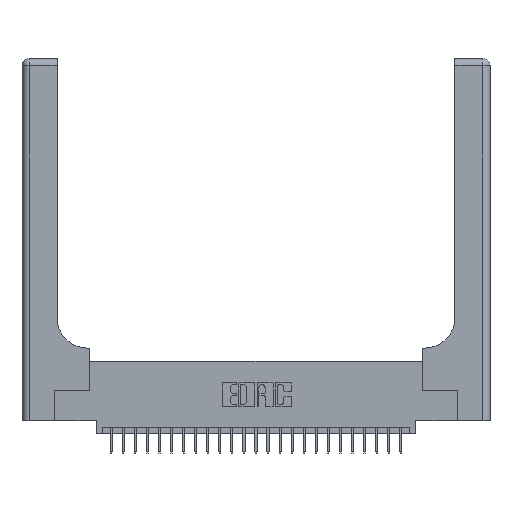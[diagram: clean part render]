
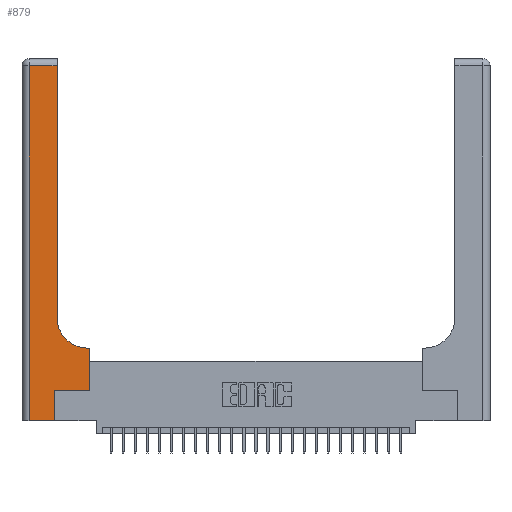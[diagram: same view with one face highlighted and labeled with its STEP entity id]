
A CAD part, top view. The second image highlights one B-rep face of the part: STEP entity #879.
In plain terms, the highlighted planar face has unit normal (0, 0, 1).
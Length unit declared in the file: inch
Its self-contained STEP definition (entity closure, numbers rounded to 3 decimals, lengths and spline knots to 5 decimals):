
#656 = DIRECTION ( 'NONE',  ( 0., 1., 0. ) ) ;
#753 = ORIENTED_EDGE ( 'NONE', *, *, #13898, .T. ) ;
#775 = CARTESIAN_POINT ( 'NONE',  ( 0.5415, 0.85, 0.37 ) ) ;
#879 = ADVANCED_FACE ( 'NONE', ( #22468 ), #5520, .F. ) ;
#1070 = CARTESIAN_POINT ( 'NONE',  ( 0.2915, 2.94, 0.37 ) ) ;
#1868 = EDGE_CURVE ( 'NONE', #20469, #19762, #23070, .T. ) ;
#2845 = ORIENTED_EDGE ( 'NONE', *, *, #1868, .T. ) ;
#3010 = DIRECTION ( 'NONE',  ( 1., 0., 0. ) ) ;
#3259 = CARTESIAN_POINT ( 'NONE',  ( 0.269, 0.25, 0.37 ) ) ;
#3260 = CARTESIAN_POINT ( 'NONE',  ( 0.06, 2.94, 0.37 ) ) ;
#3506 = VECTOR ( 'NONE', #7348, 39.37008 ) ;
#4232 = EDGE_CURVE ( 'NONE', #21338, #11425, #9016, .T. ) ;
#4627 = EDGE_CURVE ( 'NONE', #11385, #20416, #11005, .T. ) ;
#4707 = EDGE_CURVE ( 'NONE', #4932, #11385, #24856, .T. ) ;
#4847 = LINE ( 'NONE', #16054, #20921 ) ;
#4932 = VERTEX_POINT ( 'NONE', #3260 ) ;
#5264 = DIRECTION ( 'NONE',  ( -1., 0., 0. ) ) ;
#5421 = DIRECTION ( 'NONE',  ( 0., 0., -1. ) ) ;
#5474 = CARTESIAN_POINT ( 'NONE',  ( 0., 3., 0.37 ) ) ;
#5520 = PLANE ( 'NONE',  #12516 ) ;
#5882 = LINE ( 'NONE', #26482, #6572 ) ;
#6572 = VECTOR ( 'NONE', #14199, 39.37008 ) ;
#7348 = DIRECTION ( 'NONE',  ( 0., 1., 0. ) ) ;
#7448 = CARTESIAN_POINT ( 'NONE',  ( 0.5585, 0.25, 0.37 ) ) ;
#8783 = DIRECTION ( 'NONE',  ( 0., -1., 0. ) ) ;
#8971 = ORIENTED_EDGE ( 'NONE', *, *, #26906, .T. ) ;
#8988 = VECTOR ( 'NONE', #8783, 39.37008 ) ;
#9016 = LINE ( 'NONE', #17644, #13956 ) ;
#10276 = CARTESIAN_POINT ( 'NONE',  ( 0.269, 0., 0.37 ) ) ;
#10297 = VERTEX_POINT ( 'NONE', #3259 ) ;
#10330 = VECTOR ( 'NONE', #12772, 39.37008 ) ;
#10496 = CARTESIAN_POINT ( 'NONE',  ( 0.5415, 0.6, 0.37 ) ) ;
#10665 = CARTESIAN_POINT ( 'NONE',  ( 0., 0., 0.37 ) ) ;
#11005 = LINE ( 'NONE', #10665, #10330 ) ;
#11385 = VERTEX_POINT ( 'NONE', #11789 ) ;
#11425 = VERTEX_POINT ( 'NONE', #1070 ) ;
#11468 = DIRECTION ( 'NONE',  ( 1., 0., 0. ) ) ;
#11789 = CARTESIAN_POINT ( 'NONE',  ( 0.06, 0., 0.37 ) ) ;
#11911 = CARTESIAN_POINT ( 'NONE',  ( 0.269, 0.25, 0.37 ) ) ;
#12283 = ORIENTED_EDGE ( 'NONE', *, *, #24814, .T. ) ;
#12516 = AXIS2_PLACEMENT_3D ( 'NONE', #5474, #5421, #5264 ) ;
#12772 = DIRECTION ( 'NONE',  ( 1., 0., 0. ) ) ;
#13276 = ORIENTED_EDGE ( 'NONE', *, *, #4232, .T. ) ;
#13439 = VECTOR ( 'NONE', #17979, 39.37008 ) ;
#13716 = CARTESIAN_POINT ( 'NONE',  ( 0.2915, 0.85, 0.37 ) ) ;
#13767 = CIRCLE ( 'NONE', #20720, 0.25 ) ;
#13782 = EDGE_CURVE ( 'NONE', #24754, #20469, #25145, .T. ) ;
#13794 = VECTOR ( 'NONE', #11468, 39.37008 ) ;
#13898 = EDGE_CURVE ( 'NONE', #20416, #10297, #5882, .T. ) ;
#13956 = VECTOR ( 'NONE', #656, 39.37008 ) ;
#14199 = DIRECTION ( 'NONE',  ( 0., 1., 0. ) ) ;
#14247 = ORIENTED_EDGE ( 'NONE', *, *, #25285, .T. ) ;
#14427 = LINE ( 'NONE', #11911, #13794 ) ;
#15768 = DIRECTION ( 'NONE',  ( 0., 0., -1. ) ) ;
#16054 = CARTESIAN_POINT ( 'NONE',  ( 0., 2.94, 0.37 ) ) ;
#17168 = CARTESIAN_POINT ( 'NONE',  ( 0.5585, 0.6, 0.37 ) ) ;
#17644 = CARTESIAN_POINT ( 'NONE',  ( 0.2915, 3., 0.37 ) ) ;
#17979 = DIRECTION ( 'NONE',  ( -1., 0., 0. ) ) ;
#18041 = CARTESIAN_POINT ( 'NONE',  ( 0.2915, 0.6, 0.37 ) ) ;
#18407 = ORIENTED_EDGE ( 'NONE', *, *, #13782, .T. ) ;
#19149 = CARTESIAN_POINT ( 'NONE',  ( 0.06, 3., 0.37 ) ) ;
#19566 = CARTESIAN_POINT ( 'NONE',  ( 0.5585, 0.25, 0.37 ) ) ;
#19762 = VERTEX_POINT ( 'NONE', #10496 ) ;
#20016 = ORIENTED_EDGE ( 'NONE', *, *, #4707, .T. ) ;
#20349 = EDGE_LOOP ( 'NONE', ( #13276, #8971, #20016, #21308, #753, #12283, #18407, #2845, #14247 ) ) ;
#20416 = VERTEX_POINT ( 'NONE', #10276 ) ;
#20469 = VERTEX_POINT ( 'NONE', #17168 ) ;
#20720 = AXIS2_PLACEMENT_3D ( 'NONE', #775, #15768, #3010 ) ;
#20921 = VECTOR ( 'NONE', #22158, 39.37008 ) ;
#21308 = ORIENTED_EDGE ( 'NONE', *, *, #4627, .T. ) ;
#21338 = VERTEX_POINT ( 'NONE', #13716 ) ;
#22158 = DIRECTION ( 'NONE',  ( -1., 0., 0. ) ) ;
#22468 = FACE_OUTER_BOUND ( 'NONE', #20349, .T. ) ;
#23070 = LINE ( 'NONE', #18041, #13439 ) ;
#24754 = VERTEX_POINT ( 'NONE', #19566 ) ;
#24814 = EDGE_CURVE ( 'NONE', #10297, #24754, #14427, .T. ) ;
#24856 = LINE ( 'NONE', #19149, #8988 ) ;
#25145 = LINE ( 'NONE', #7448, #3506 ) ;
#25285 = EDGE_CURVE ( 'NONE', #19762, #21338, #13767, .T. ) ;
#26482 = CARTESIAN_POINT ( 'NONE',  ( 0.269, 0., 0.37 ) ) ;
#26906 = EDGE_CURVE ( 'NONE', #11425, #4932, #4847, .T. ) ;
